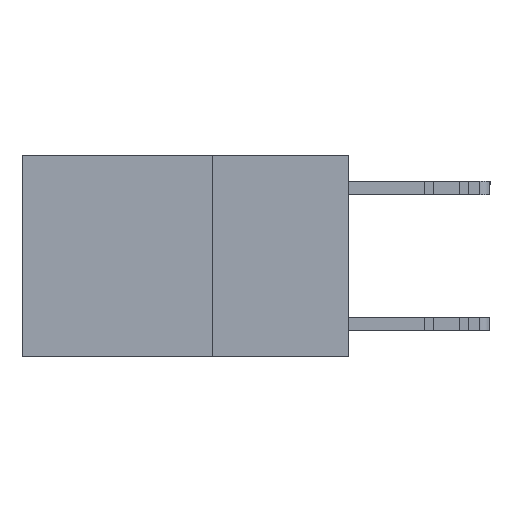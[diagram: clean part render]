
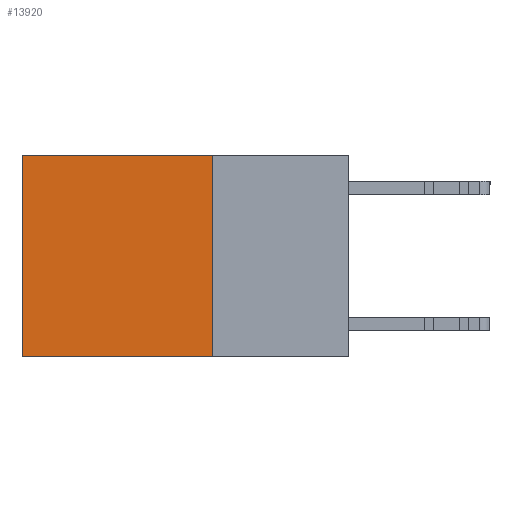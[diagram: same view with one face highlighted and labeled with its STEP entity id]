
A CAD part, left-side view. The second image highlights one B-rep face of the part: STEP entity #13920.
In plain terms, the highlighted planar face has unit normal (-1, 0, 0).
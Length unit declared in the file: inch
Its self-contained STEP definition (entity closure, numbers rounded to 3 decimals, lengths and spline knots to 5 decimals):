
#159 = CARTESIAN_POINT ( 'NONE',  ( 0.2625, 0.6, 0. ) ) ;
#552 = ORIENTED_EDGE ( 'NONE', *, *, #5865, .F. ) ;
#1233 = VERTEX_POINT ( 'NONE', #14410 ) ;
#2695 = ORIENTED_EDGE ( 'NONE', *, *, #30828, .F. ) ;
#3799 = FACE_OUTER_BOUND ( 'NONE', #21728, .T. ) ;
#4398 = VECTOR ( 'NONE', #16789, 39.37008 ) ;
#5865 = EDGE_CURVE ( 'NONE', #30378, #26752, #24546, .T. ) ;
#6285 = PLANE ( 'NONE',  #6784 ) ;
#6784 = AXIS2_PLACEMENT_3D ( 'NONE', #24147, #11581, #21836 ) ;
#6899 = DIRECTION ( 'NONE',  ( 0., 1., 0. ) ) ;
#7517 = CARTESIAN_POINT ( 'NONE',  ( 0.2625, 0.25, 0. ) ) ;
#7617 = LINE ( 'NONE', #159, #20766 ) ;
#9723 = VECTOR ( 'NONE', #6899, 39.37008 ) ;
#11006 = ORIENTED_EDGE ( 'NONE', *, *, #23131, .T. ) ;
#11581 = DIRECTION ( 'NONE',  ( 1., 0., 0. ) ) ;
#12730 = ORIENTED_EDGE ( 'NONE', *, *, #21966, .T. ) ;
#13920 = ADVANCED_FACE ( 'NONE', ( #3799 ), #6285, .F. ) ;
#14410 = CARTESIAN_POINT ( 'NONE',  ( 0.2625, 0.6, 0. ) ) ;
#16789 = DIRECTION ( 'NONE',  ( 0., 0., -1. ) ) ;
#17108 = VERTEX_POINT ( 'NONE', #31861 ) ;
#17622 = CARTESIAN_POINT ( 'NONE',  ( 0.2625, 0.25, 0. ) ) ;
#20673 = DIRECTION ( 'NONE',  ( 0., 0., -1. ) ) ;
#20766 = VECTOR ( 'NONE', #20673, 39.37008 ) ;
#21394 = VECTOR ( 'NONE', #31978, 39.37008 ) ;
#21727 = LINE ( 'NONE', #21882, #21394 ) ;
#21728 = EDGE_LOOP ( 'NONE', ( #11006, #2695, #552, #12730 ) ) ;
#21836 = DIRECTION ( 'NONE',  ( 0., 0., -1. ) ) ;
#21882 = CARTESIAN_POINT ( 'NONE',  ( 0.2625, 0.25, -0.37 ) ) ;
#21966 = EDGE_CURVE ( 'NONE', #30378, #1233, #22266, .T. ) ;
#22266 = LINE ( 'NONE', #17622, #9723 ) ;
#23131 = EDGE_CURVE ( 'NONE', #1233, #17108, #7617, .T. ) ;
#24147 = CARTESIAN_POINT ( 'NONE',  ( 0.2625, 0.25, 0. ) ) ;
#24546 = LINE ( 'NONE', #28868, #4398 ) ;
#26752 = VERTEX_POINT ( 'NONE', #32589 ) ;
#28868 = CARTESIAN_POINT ( 'NONE',  ( 0.2625, 0.25, 0. ) ) ;
#30378 = VERTEX_POINT ( 'NONE', #7517 ) ;
#30828 = EDGE_CURVE ( 'NONE', #26752, #17108, #21727, .T. ) ;
#31861 = CARTESIAN_POINT ( 'NONE',  ( 0.2625, 0.6, -0.37 ) ) ;
#31978 = DIRECTION ( 'NONE',  ( 0., 1., 0. ) ) ;
#32589 = CARTESIAN_POINT ( 'NONE',  ( 0.2625, 0.25, -0.37 ) ) ;
